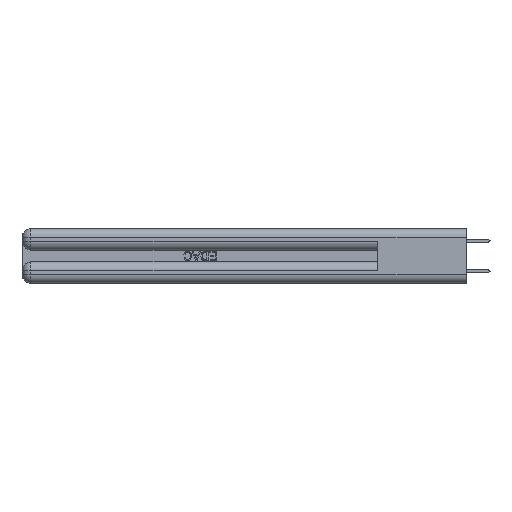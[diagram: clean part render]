
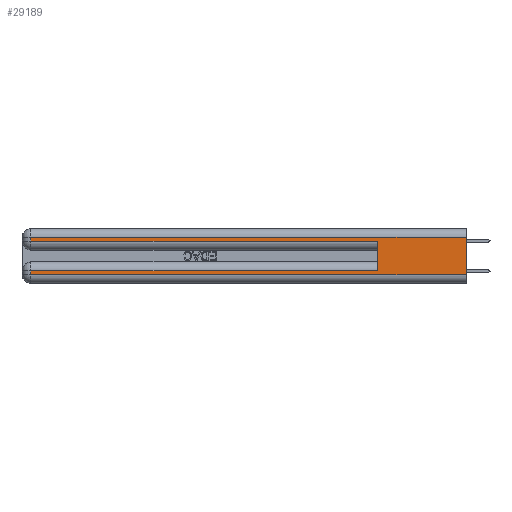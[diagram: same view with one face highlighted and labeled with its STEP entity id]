
A CAD part, left-side view. The second image highlights one B-rep face of the part: STEP entity #29189.
In plain terms, the highlighted planar face has unit normal (-1, 0, 0).
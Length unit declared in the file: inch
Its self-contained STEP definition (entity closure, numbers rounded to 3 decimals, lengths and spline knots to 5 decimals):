
#1529 = EDGE_CURVE ( 'NONE', #6070, #40051, #25992, .T. ) ;
#4501 = PLANE ( 'NONE',  #33060 ) ;
#5323 = FACE_OUTER_BOUND ( 'NONE', #16260, .T. ) ;
#6001 = VECTOR ( 'NONE', #10643, 39.37008 ) ;
#6070 = VERTEX_POINT ( 'NONE', #28688 ) ;
#6260 = DIRECTION ( 'NONE',  ( 0., 0., -1. ) ) ;
#6337 = LINE ( 'NONE', #44221, #45079 ) ;
#6505 = DIRECTION ( 'NONE',  ( 0., -1., 0. ) ) ;
#7905 = EDGE_CURVE ( 'NONE', #27378, #26556, #6337, .T. ) ;
#7974 = CARTESIAN_POINT ( 'NONE',  ( 0., 0., 0.37 ) ) ;
#8851 = VECTOR ( 'NONE', #16281, 39.37008 ) ;
#9576 = ORIENTED_EDGE ( 'NONE', *, *, #32486, .T. ) ;
#10052 = DIRECTION ( 'NONE',  ( 0., 1., 0. ) ) ;
#10643 = DIRECTION ( 'NONE',  ( 0., 1., 0. ) ) ;
#11647 = VERTEX_POINT ( 'NONE', #22516 ) ;
#11757 = DIRECTION ( 'NONE',  ( 0., 0., -1. ) ) ;
#12233 = DIRECTION ( 'NONE',  ( 1., 0., 0. ) ) ;
#12292 = VECTOR ( 'NONE', #6260, 39.37008 ) ;
#15030 = ORIENTED_EDGE ( 'NONE', *, *, #46893, .F. ) ;
#15568 = VECTOR ( 'NONE', #32029, 39.37008 ) ;
#16260 = EDGE_LOOP ( 'NONE', ( #15030, #36981, #17885, #9576, #28747, #23960, #22364, #43469 ) ) ;
#16281 = DIRECTION ( 'NONE',  ( 0., 0., 1. ) ) ;
#17885 = ORIENTED_EDGE ( 'NONE', *, *, #45116, .T. ) ;
#18470 = LINE ( 'NONE', #32345, #15568 ) ;
#18501 = CARTESIAN_POINT ( 'NONE',  ( 0., 0., 0.06 ) ) ;
#19088 = LINE ( 'NONE', #22012, #47875 ) ;
#19732 = DIRECTION ( 'NONE',  ( 0., 0., -1. ) ) ;
#22012 = CARTESIAN_POINT ( 'NONE',  ( 0., 0., 0.285 ) ) ;
#22070 = CARTESIAN_POINT ( 'NONE',  ( 0., 2.94, 0.285 ) ) ;
#22364 = ORIENTED_EDGE ( 'NONE', *, *, #36527, .T. ) ;
#22516 = CARTESIAN_POINT ( 'NONE',  ( 0., 2.94, 0.085 ) ) ;
#22897 = LINE ( 'NONE', #43640, #12292 ) ;
#23064 = CARTESIAN_POINT ( 'NONE',  ( 0., 2.94, 0.06 ) ) ;
#23960 = ORIENTED_EDGE ( 'NONE', *, *, #40015, .T. ) ;
#25009 = CARTESIAN_POINT ( 'NONE',  ( 0., 0.6, 0.285 ) ) ;
#25992 = LINE ( 'NONE', #29373, #6001 ) ;
#26054 = VECTOR ( 'NONE', #10052, 39.37008 ) ;
#26556 = VERTEX_POINT ( 'NONE', #18501 ) ;
#27378 = VERTEX_POINT ( 'NONE', #23064 ) ;
#27788 = CARTESIAN_POINT ( 'NONE',  ( 0., 0.6, 0.145 ) ) ;
#28314 = LINE ( 'NONE', #42516, #34151 ) ;
#28688 = CARTESIAN_POINT ( 'NONE',  ( 0., 0., 0.31 ) ) ;
#28747 = ORIENTED_EDGE ( 'NONE', *, *, #35368, .F. ) ;
#29189 = ADVANCED_FACE ( 'NONE', ( #5323 ), #4501, .F. ) ;
#29373 = CARTESIAN_POINT ( 'NONE',  ( 0., 0., 0.31 ) ) ;
#29584 = CARTESIAN_POINT ( 'NONE',  ( 0., 2.94, 0.31 ) ) ;
#29983 = VERTEX_POINT ( 'NONE', #22070 ) ;
#30573 = LINE ( 'NONE', #27788, #8851 ) ;
#32029 = DIRECTION ( 'NONE',  ( 0., 0., -1. ) ) ;
#32345 = CARTESIAN_POINT ( 'NONE',  ( 0., 2.94, 0.37 ) ) ;
#32486 = EDGE_CURVE ( 'NONE', #29983, #40043, #19088, .T. ) ;
#33060 = AXIS2_PLACEMENT_3D ( 'NONE', #7974, #12233, #11757 ) ;
#34151 = VECTOR ( 'NONE', #19732, 39.37008 ) ;
#35368 = EDGE_CURVE ( 'NONE', #37715, #40043, #30573, .T. ) ;
#35953 = CARTESIAN_POINT ( 'NONE',  ( 0., 0., 0.085 ) ) ;
#36527 = EDGE_CURVE ( 'NONE', #11647, #27378, #22897, .T. ) ;
#36981 = ORIENTED_EDGE ( 'NONE', *, *, #1529, .T. ) ;
#37715 = VERTEX_POINT ( 'NONE', #38970 ) ;
#38970 = CARTESIAN_POINT ( 'NONE',  ( 0., 0.6, 0.085 ) ) ;
#40015 = EDGE_CURVE ( 'NONE', #37715, #11647, #46008, .T. ) ;
#40043 = VERTEX_POINT ( 'NONE', #25009 ) ;
#40051 = VERTEX_POINT ( 'NONE', #29584 ) ;
#42516 = CARTESIAN_POINT ( 'NONE',  ( 0., 0., 0.37 ) ) ;
#43469 = ORIENTED_EDGE ( 'NONE', *, *, #7905, .T. ) ;
#43640 = CARTESIAN_POINT ( 'NONE',  ( 0., 2.94, 0.37 ) ) ;
#44221 = CARTESIAN_POINT ( 'NONE',  ( 0., 0., 0.06 ) ) ;
#45079 = VECTOR ( 'NONE', #6505, 39.37008 ) ;
#45116 = EDGE_CURVE ( 'NONE', #40051, #29983, #18470, .T. ) ;
#46008 = LINE ( 'NONE', #35953, #26054 ) ;
#46893 = EDGE_CURVE ( 'NONE', #6070, #26556, #28314, .T. ) ;
#47875 = VECTOR ( 'NONE', #47947, 39.37008 ) ;
#47947 = DIRECTION ( 'NONE',  ( 0., -1., 0. ) ) ;
